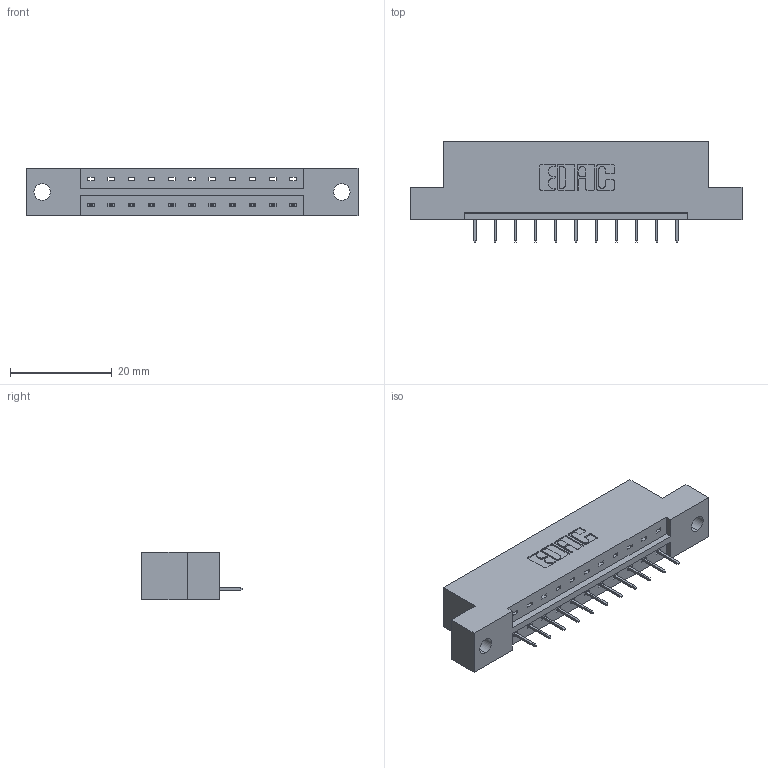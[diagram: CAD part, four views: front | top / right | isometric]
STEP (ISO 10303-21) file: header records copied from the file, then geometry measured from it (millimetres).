
FILE_DESCRIPTION (( 'STEP AP203' ), '1' );
FILE_NAME ('833-011-524-102.STEP', '2020-05-30T19:38:35', ( '' ), ( '' ), 'SwSTEP 2.0', 'SolidWorks 2020', '' );
FILE_SCHEMA (( 'CONFIG_CONTROL_DESIGN' ));
Length unit declared in the file: inch
Products named in the file (3): 833-011-524-102; 833 Part_Flush - .128 Dia; 345-292-001_345-293-124
Assembly tree (12 placements, depth 2):
  833-011-524-102
    833 Part_Flush - .128 Dia
    345-292-001_345-293-124  x11
Bounding box: 65.13 x 19.69 x 9.4 mm (x, y, z)
Volume: 6206.7 mm3; surface area: 6091.1 mm2
Topology: 12 solids, 12 shells, 796 faces, 2291 edges, 1482 vertices
Faces by surface type: plane 598, cylinder 198
Entity records: 10811 total; most frequent: CARTESIAN_POINT 1875, ORIENTED_EDGE 1822, DIRECTION 1645, EDGE_CURVE 911, VECTOR 787, LINE 787, VERTEX_POINT 602, AXIS2_PLACEMENT_3D 429
